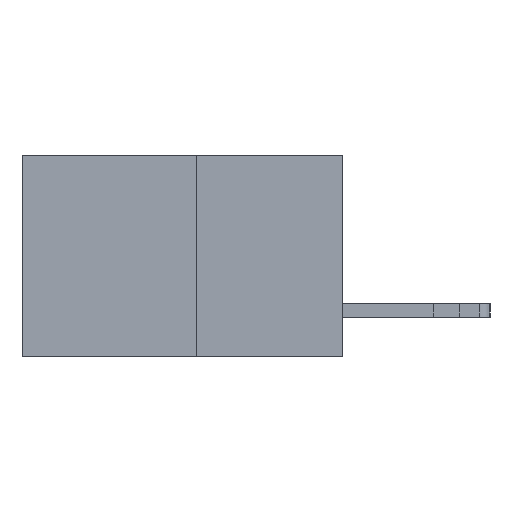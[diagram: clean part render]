
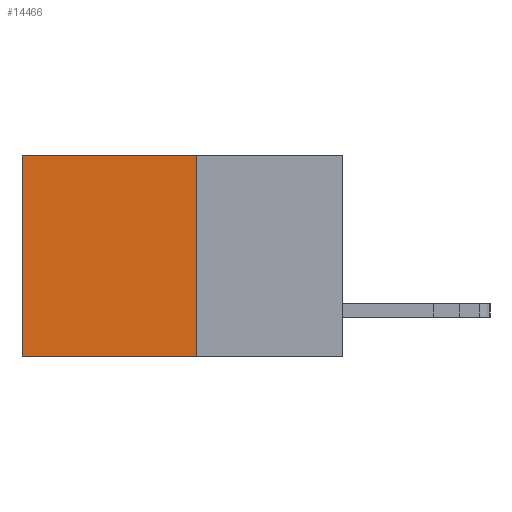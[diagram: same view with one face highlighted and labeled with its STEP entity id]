
A CAD part, left-side view. The second image highlights one B-rep face of the part: STEP entity #14466.
In plain terms, the highlighted planar face has unit normal (-1, 0, 0).
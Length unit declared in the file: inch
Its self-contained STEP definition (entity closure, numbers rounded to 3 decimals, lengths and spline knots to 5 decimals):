
#24 = CARTESIAN_POINT ( 'NONE',  ( 0.277, 0.27, 0. ) ) ;
#163 = LINE ( 'NONE', #24, #18084 ) ;
#1420 = CARTESIAN_POINT ( 'NONE',  ( 0.277, 0.27, -0.37 ) ) ;
#1946 = FACE_OUTER_BOUND ( 'NONE', #19749, .T. ) ;
#2053 = VECTOR ( 'NONE', #13231, 39.37008 ) ;
#2165 = DIRECTION ( 'NONE',  ( 0., 1., 0. ) ) ;
#2225 = VECTOR ( 'NONE', #8139, 39.37008 ) ;
#4293 = EDGE_CURVE ( 'NONE', #10472, #11979, #14157, .T. ) ;
#5855 = CARTESIAN_POINT ( 'NONE',  ( 0.277, 0.27, -0.37 ) ) ;
#7974 = CARTESIAN_POINT ( 'NONE',  ( 0.277, 0.27, -0.37 ) ) ;
#8139 = DIRECTION ( 'NONE',  ( 0., 1., 0. ) ) ;
#8146 = EDGE_CURVE ( 'NONE', #22300, #11979, #9974, .T. ) ;
#8198 = DIRECTION ( 'NONE',  ( 1., 0., 0. ) ) ;
#8717 = LINE ( 'NONE', #10976, #2053 ) ;
#9974 = LINE ( 'NONE', #12231, #21293 ) ;
#10319 = CARTESIAN_POINT ( 'NONE',  ( 0.277, 0.27, 0. ) ) ;
#10472 = VERTEX_POINT ( 'NONE', #7974 ) ;
#10830 = CARTESIAN_POINT ( 'NONE',  ( 0.277, 0.59, -0.37 ) ) ;
#10976 = CARTESIAN_POINT ( 'NONE',  ( 0.277, 0.27, -0.37 ) ) ;
#11665 = ORIENTED_EDGE ( 'NONE', *, *, #20170, .T. ) ;
#11979 = VERTEX_POINT ( 'NONE', #10830 ) ;
#12231 = CARTESIAN_POINT ( 'NONE',  ( 0.277, 0.59, -0.37 ) ) ;
#12546 = CARTESIAN_POINT ( 'NONE',  ( 0.277, 0.59, 0. ) ) ;
#13231 = DIRECTION ( 'NONE',  ( 0., 0., -1. ) ) ;
#14065 = ORIENTED_EDGE ( 'NONE', *, *, #4293, .F. ) ;
#14157 = LINE ( 'NONE', #5855, #2225 ) ;
#14466 = ADVANCED_FACE ( 'NONE', ( #1946 ), #21693, .F. ) ;
#15688 = ORIENTED_EDGE ( 'NONE', *, *, #26927, .F. ) ;
#18084 = VECTOR ( 'NONE', #2165, 39.37008 ) ;
#19350 = VERTEX_POINT ( 'NONE', #10319 ) ;
#19749 = EDGE_LOOP ( 'NONE', ( #28038, #14065, #15688, #11665 ) ) ;
#20170 = EDGE_CURVE ( 'NONE', #19350, #22300, #163, .T. ) ;
#21293 = VECTOR ( 'NONE', #27987, 39.37008 ) ;
#21693 = PLANE ( 'NONE',  #25128 ) ;
#22300 = VERTEX_POINT ( 'NONE', #12546 ) ;
#23964 = DIRECTION ( 'NONE',  ( 0., 0., -1. ) ) ;
#25128 = AXIS2_PLACEMENT_3D ( 'NONE', #1420, #8198, #23964 ) ;
#26927 = EDGE_CURVE ( 'NONE', #19350, #10472, #8717, .T. ) ;
#27987 = DIRECTION ( 'NONE',  ( 0., 0., -1. ) ) ;
#28038 = ORIENTED_EDGE ( 'NONE', *, *, #8146, .T. ) ;
